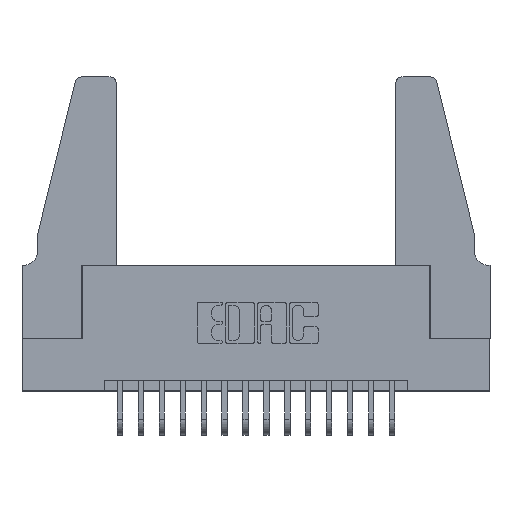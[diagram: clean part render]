
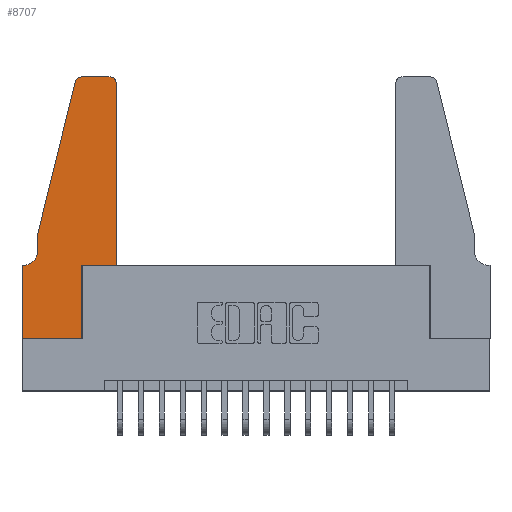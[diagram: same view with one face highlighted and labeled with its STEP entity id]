
A CAD part, top view. The second image highlights one B-rep face of the part: STEP entity #8707.
In plain terms, the highlighted planar face has unit normal (0, 0, 1).
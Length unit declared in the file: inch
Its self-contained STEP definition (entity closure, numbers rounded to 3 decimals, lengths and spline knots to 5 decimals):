
#361 = EDGE_CURVE ( 'NONE', #5971, #1744, #14879, .T. ) ;
#666 = CARTESIAN_POINT ( 'NONE',  ( 0.0055, 0.42, 0.37 ) ) ;
#837 = DIRECTION ( 'NONE',  ( 0., -1., 0. ) ) ;
#880 = FACE_OUTER_BOUND ( 'NONE', #9443, .T. ) ;
#957 = CARTESIAN_POINT ( 'NONE',  ( 0.4505, 1.22, 0.37 ) ) ;
#1083 = CARTESIAN_POINT ( 'NONE',  ( 0.284, 1.22, 0.37 ) ) ;
#1107 = CARTESIAN_POINT ( 'NONE',  ( 0.25487, 1.22718, 0.37 ) ) ;
#1486 = CARTESIAN_POINT ( 'NONE',  ( 0.0755, 0.42, 0.37 ) ) ;
#1540 = ORIENTED_EDGE ( 'NONE', *, *, #3852, .T. ) ;
#1578 = EDGE_CURVE ( 'NONE', #12443, #18172, #4158, .T. ) ;
#1744 = VERTEX_POINT ( 'NONE', #1107 ) ;
#2204 = DIRECTION ( 'NONE',  ( -1., 0., 0. ) ) ;
#2682 = DIRECTION ( 'NONE',  ( 1., 0., 0. ) ) ;
#2743 = CARTESIAN_POINT ( 'NONE',  ( 0.2605, 1.25, 0.37 ) ) ;
#3042 = EDGE_CURVE ( 'NONE', #7539, #4910, #14122, .T. ) ;
#3155 = VECTOR ( 'NONE', #7566, 39.37008 ) ;
#3236 = ORIENTED_EDGE ( 'NONE', *, *, #1578, .T. ) ;
#3238 = CARTESIAN_POINT ( 'NONE',  ( 0.4505, 0.35, 0.37 ) ) ;
#3545 = AXIS2_PLACEMENT_3D ( 'NONE', #666, #10872, #2204 ) ;
#3603 = VECTOR ( 'NONE', #15853, 39.37008 ) ;
#3708 = VECTOR ( 'NONE', #2682, 39.37008 ) ;
#3852 = EDGE_CURVE ( 'NONE', #18172, #7539, #14552, .T. ) ;
#4158 = LINE ( 'NONE', #3238, #3708 ) ;
#4213 = LINE ( 'NONE', #14071, #8549 ) ;
#4364 = AXIS2_PLACEMENT_3D ( 'NONE', #1083, #17328, #4674 ) ;
#4674 = DIRECTION ( 'NONE',  ( 1., 0., 0. ) ) ;
#4910 = VERTEX_POINT ( 'NONE', #5643 ) ;
#4946 = VERTEX_POINT ( 'NONE', #12441 ) ;
#5009 = EDGE_CURVE ( 'NONE', #4946, #10648, #16295, .T. ) ;
#5473 = CARTESIAN_POINT ( 'NONE',  ( 0.2865, 0.35, 0.37 ) ) ;
#5580 = ORIENTED_EDGE ( 'NONE', *, *, #15334, .T. ) ;
#5595 = VECTOR ( 'NONE', #12823, 39.37008 ) ;
#5643 = CARTESIAN_POINT ( 'NONE',  ( 0.4205, 1.25, 0.37 ) ) ;
#5879 = CARTESIAN_POINT ( 'NONE',  ( 0.4205, 1.22, 0.37 ) ) ;
#5920 = ORIENTED_EDGE ( 'NONE', *, *, #11224, .T. ) ;
#5971 = VERTEX_POINT ( 'NONE', #17598 ) ;
#6076 = VECTOR ( 'NONE', #837, 39.37008 ) ;
#6104 = CARTESIAN_POINT ( 'NONE',  ( 0.4505, 0.35, 0.37 ) ) ;
#6231 = ORIENTED_EDGE ( 'NONE', *, *, #3042, .T. ) ;
#6298 = LINE ( 'NONE', #2743, #12464 ) ;
#6776 = CARTESIAN_POINT ( 'NONE',  ( 0.0755, 0.5, 0.37 ) ) ;
#6964 = ORIENTED_EDGE ( 'NONE', *, *, #13141, .T. ) ;
#7061 = CARTESIAN_POINT ( 'NONE',  ( 0.0055, 0.35, 0.37 ) ) ;
#7338 = DIRECTION ( 'NONE',  ( 1., 0., 0. ) ) ;
#7485 = EDGE_CURVE ( 'NONE', #17678, #13861, #10314, .T. ) ;
#7496 = LINE ( 'NONE', #14466, #3603 ) ;
#7539 = VERTEX_POINT ( 'NONE', #957 ) ;
#7566 = DIRECTION ( 'NONE',  ( 0., 1., 0. ) ) ;
#7598 = EDGE_CURVE ( 'NONE', #1744, #17678, #4213, .T. ) ;
#8549 = VECTOR ( 'NONE', #9930, 39.37008 ) ;
#8707 = ADVANCED_FACE ( 'NONE', ( #880 ), #10427, .T. ) ;
#9091 = DIRECTION ( 'NONE',  ( 1., 0., 0. ) ) ;
#9443 = EDGE_LOOP ( 'NONE', ( #6964, #18489, #18001, #14910, #5580, #18393, #12577, #15771, #5920, #3236, #1540, #6231 ) ) ;
#9453 = CARTESIAN_POINT ( 'NONE',  ( 0.0755, 0.5, 0.37 ) ) ;
#9585 = VERTEX_POINT ( 'NONE', #9600 ) ;
#9600 = CARTESIAN_POINT ( 'NONE',  ( 0.2865, 0., 0.37 ) ) ;
#9721 = VERTEX_POINT ( 'NONE', #7061 ) ;
#9930 = DIRECTION ( 'NONE',  ( -0.239, -0.971, 0. ) ) ;
#10042 = CARTESIAN_POINT ( 'NONE',  ( 0., 0., 0.37 ) ) ;
#10314 = LINE ( 'NONE', #6776, #6076 ) ;
#10427 = PLANE ( 'NONE',  #13963 ) ;
#10648 = VERTEX_POINT ( 'NONE', #17660 ) ;
#10872 = DIRECTION ( 'NONE',  ( 0., 0., -1. ) ) ;
#11224 = EDGE_CURVE ( 'NONE', #9585, #12443, #15159, .T. ) ;
#11454 = EDGE_CURVE ( 'NONE', #9721, #4946, #7496, .T. ) ;
#11884 = VECTOR ( 'NONE', #16730, 39.37008 ) ;
#12441 = CARTESIAN_POINT ( 'NONE',  ( 0., 0.35, 0.37 ) ) ;
#12443 = VERTEX_POINT ( 'NONE', #16807 ) ;
#12464 = VECTOR ( 'NONE', #15498, 39.37008 ) ;
#12577 = ORIENTED_EDGE ( 'NONE', *, *, #5009, .T. ) ;
#12607 = CARTESIAN_POINT ( 'NONE',  ( 0., 0., 0.37 ) ) ;
#12823 = DIRECTION ( 'NONE',  ( 1., 0., 0. ) ) ;
#13141 = EDGE_CURVE ( 'NONE', #4910, #5971, #6298, .T. ) ;
#13225 = CARTESIAN_POINT ( 'NONE',  ( 0., 0.35, 0.37 ) ) ;
#13861 = VERTEX_POINT ( 'NONE', #1486 ) ;
#13963 = AXIS2_PLACEMENT_3D ( 'NONE', #13225, #17426, #9091 ) ;
#14028 = DIRECTION ( 'NONE',  ( 0., -1., 0. ) ) ;
#14071 = CARTESIAN_POINT ( 'NONE',  ( 0.0755, 0.5, 0.37 ) ) ;
#14122 = CIRCLE ( 'NONE', #14271, 0.03 ) ;
#14271 = AXIS2_PLACEMENT_3D ( 'NONE', #5879, #15712, #7338 ) ;
#14462 = EDGE_CURVE ( 'NONE', #10648, #9585, #16390, .T. ) ;
#14466 = CARTESIAN_POINT ( 'NONE',  ( 0.0755, 0.35, 0.37 ) ) ;
#14552 = LINE ( 'NONE', #6104, #3155 ) ;
#14879 = CIRCLE ( 'NONE', #4364, 0.03 ) ;
#14910 = ORIENTED_EDGE ( 'NONE', *, *, #7485, .T. ) ;
#15159 = LINE ( 'NONE', #5473, #11884 ) ;
#15334 = EDGE_CURVE ( 'NONE', #13861, #9721, #15893, .T. ) ;
#15400 = VECTOR ( 'NONE', #14028, 39.37008 ) ;
#15498 = DIRECTION ( 'NONE',  ( -1., 0., 0. ) ) ;
#15712 = DIRECTION ( 'NONE',  ( 0., 0., 1. ) ) ;
#15771 = ORIENTED_EDGE ( 'NONE', *, *, #14462, .T. ) ;
#15853 = DIRECTION ( 'NONE',  ( -1., 0., 0. ) ) ;
#15893 = CIRCLE ( 'NONE', #3545, 0.07 ) ;
#16295 = LINE ( 'NONE', #12607, #15400 ) ;
#16331 = CARTESIAN_POINT ( 'NONE',  ( 0.4505, 0.35, 0.37 ) ) ;
#16390 = LINE ( 'NONE', #10042, #5595 ) ;
#16730 = DIRECTION ( 'NONE',  ( 0., 1., 0. ) ) ;
#16807 = CARTESIAN_POINT ( 'NONE',  ( 0.2865, 0.35, 0.37 ) ) ;
#17328 = DIRECTION ( 'NONE',  ( 0., 0., 1. ) ) ;
#17426 = DIRECTION ( 'NONE',  ( 0., 0., 1. ) ) ;
#17598 = CARTESIAN_POINT ( 'NONE',  ( 0.284, 1.25, 0.37 ) ) ;
#17660 = CARTESIAN_POINT ( 'NONE',  ( 0., 0., 0.37 ) ) ;
#17678 = VERTEX_POINT ( 'NONE', #9453 ) ;
#18001 = ORIENTED_EDGE ( 'NONE', *, *, #7598, .T. ) ;
#18172 = VERTEX_POINT ( 'NONE', #16331 ) ;
#18393 = ORIENTED_EDGE ( 'NONE', *, *, #11454, .T. ) ;
#18489 = ORIENTED_EDGE ( 'NONE', *, *, #361, .T. ) ;
